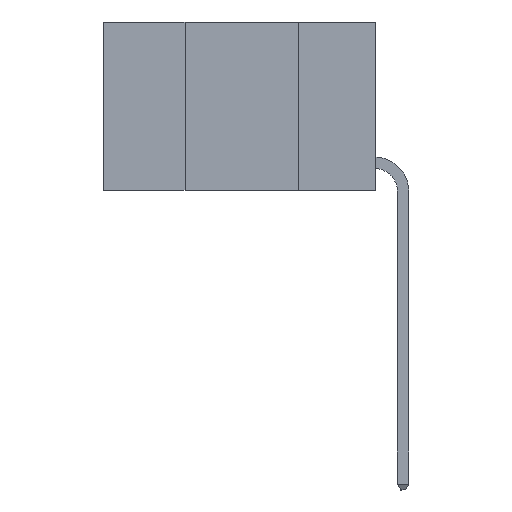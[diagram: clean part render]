
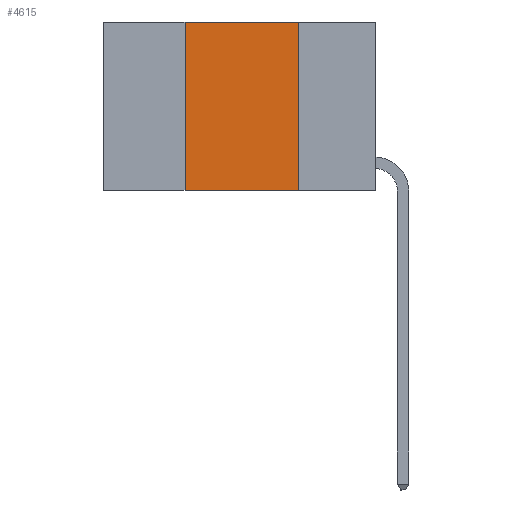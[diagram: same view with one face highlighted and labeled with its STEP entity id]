
A CAD part, left-side view. The second image highlights one B-rep face of the part: STEP entity #4615.
In plain terms, the highlighted planar face has unit normal (-1, 0, 0).
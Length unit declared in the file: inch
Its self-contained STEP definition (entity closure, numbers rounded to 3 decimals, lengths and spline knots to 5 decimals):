
#85 = VERTEX_POINT ( 'NONE', #8126 ) ;
#237 = DIRECTION ( 'NONE',  ( 0., 0., -1. ) ) ;
#1029 = CARTESIAN_POINT ( 'NONE',  ( 0., 0.42, -0.37 ) ) ;
#1099 = VECTOR ( 'NONE', #9056, 39.37008 ) ;
#1232 = CARTESIAN_POINT ( 'NONE',  ( 0., 0.17, 0. ) ) ;
#1589 = EDGE_CURVE ( 'NONE', #10616, #8876, #14227, .T. ) ;
#1681 = LINE ( 'NONE', #13476, #7486 ) ;
#2906 = DIRECTION ( 'NONE',  ( 0., 0., 1. ) ) ;
#3316 = VERTEX_POINT ( 'NONE', #10867 ) ;
#3495 = FACE_OUTER_BOUND ( 'NONE', #8108, .T. ) ;
#4490 = CARTESIAN_POINT ( 'NONE',  ( 0., 0.6, 0. ) ) ;
#4615 = ADVANCED_FACE ( 'NONE', ( #3495 ), #6684, .F. ) ;
#4978 = ORIENTED_EDGE ( 'NONE', *, *, #6504, .F. ) ;
#5094 = ORIENTED_EDGE ( 'NONE', *, *, #1589, .T. ) ;
#5448 = ORIENTED_EDGE ( 'NONE', *, *, #7946, .F. ) ;
#5887 = LINE ( 'NONE', #1232, #11838 ) ;
#6504 = EDGE_CURVE ( 'NONE', #3316, #8876, #5887, .T. ) ;
#6684 = PLANE ( 'NONE',  #7865 ) ;
#7009 = CARTESIAN_POINT ( 'NONE',  ( 0., 0.6, -0.37 ) ) ;
#7486 = VECTOR ( 'NONE', #2906, 39.37008 ) ;
#7865 = AXIS2_PLACEMENT_3D ( 'NONE', #4490, #10190, #8051 ) ;
#7946 = EDGE_CURVE ( 'NONE', #10616, #85, #1681, .T. ) ;
#8051 = DIRECTION ( 'NONE',  ( 0., 0., -1. ) ) ;
#8108 = EDGE_LOOP ( 'NONE', ( #4978, #13562, #5448, #5094 ) ) ;
#8126 = CARTESIAN_POINT ( 'NONE',  ( 0., 0.42, 0. ) ) ;
#8876 = VERTEX_POINT ( 'NONE', #9113 ) ;
#9056 = DIRECTION ( 'NONE',  ( 0., -1., 0. ) ) ;
#9113 = CARTESIAN_POINT ( 'NONE',  ( 0., 0.17, -0.37 ) ) ;
#9759 = EDGE_CURVE ( 'NONE', #85, #3316, #11260, .T. ) ;
#10190 = DIRECTION ( 'NONE',  ( 1., 0., 0. ) ) ;
#10616 = VERTEX_POINT ( 'NONE', #1029 ) ;
#10867 = CARTESIAN_POINT ( 'NONE',  ( 0., 0.17, 0. ) ) ;
#11260 = LINE ( 'NONE', #13841, #1099 ) ;
#11642 = VECTOR ( 'NONE', #14086, 39.37008 ) ;
#11838 = VECTOR ( 'NONE', #237, 39.37008 ) ;
#13476 = CARTESIAN_POINT ( 'NONE',  ( 0., 0.42, 0. ) ) ;
#13562 = ORIENTED_EDGE ( 'NONE', *, *, #9759, .F. ) ;
#13841 = CARTESIAN_POINT ( 'NONE',  ( 0., 0.6, 0. ) ) ;
#14086 = DIRECTION ( 'NONE',  ( 0., -1., 0. ) ) ;
#14227 = LINE ( 'NONE', #7009, #11642 ) ;
